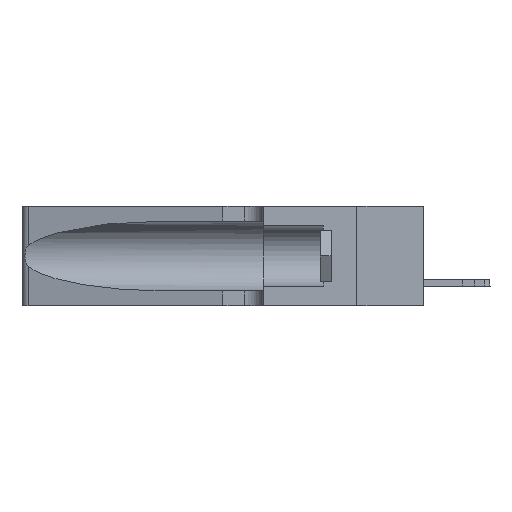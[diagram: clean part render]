
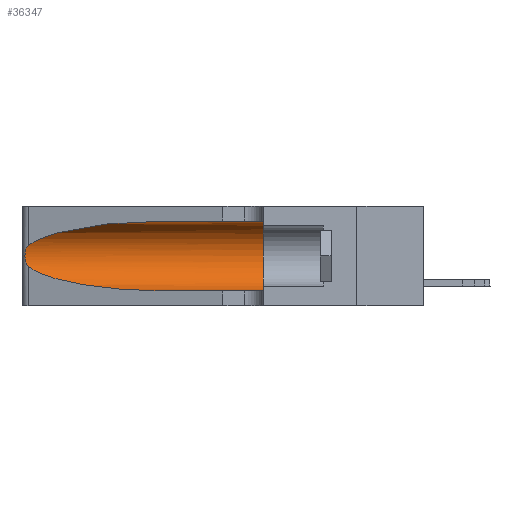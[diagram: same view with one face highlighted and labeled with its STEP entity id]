
A CAD part, left-side view. The second image highlights one B-rep face of the part: STEP entity #36347.
In plain terms, the highlighted cylindrical face has radius 3.308 mm (diameter 6.617 mm), a partial arc.
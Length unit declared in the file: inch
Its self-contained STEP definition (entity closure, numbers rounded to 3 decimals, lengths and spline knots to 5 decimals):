
#1433 = VECTOR ( 'NONE', #16997, 39.37008 ) ;
#1900 = ORIENTED_EDGE ( 'NONE', *, *, #30829, .F. ) ;
#3373 =( BOUNDED_CURVE ( )  B_SPLINE_CURVE ( 3, ( #14311, #23083, #34275, #22967 ),
 .UNSPECIFIED., .F., .F. ) 
 B_SPLINE_CURVE_WITH_KNOTS ( ( 4, 4 ),
 ( 1.5708, 2.84003 ),
 .UNSPECIFIED. ) 
 CURVE ( )  GEOMETRIC_REPRESENTATION_ITEM ( )  RATIONAL_B_SPLINE_CURVE ( ( 1., 0.87, 0.87, 1. ) ) 
 REPRESENTATION_ITEM ( '' )  );
#4114 = LINE ( 'NONE', #8895, #1433 ) ;
#4360 = CARTESIAN_POINT ( 'NONE',  ( 0.25639, 1.23184, 0.21858 ) ) ;
#4485 = CARTESIAN_POINT ( 'NONE',  ( 0.26075, 1.23896, 0.178 ) ) ;
#4694 = EDGE_CURVE ( 'NONE', #17199, #26774, #3373, .T. ) ;
#6088 = B_SPLINE_CURVE_WITH_KNOTS ( 'NONE', 3,
 ( #10452, #27189, #4360, #35996, #30304, #21318, #24179, #4485, #7190, #27065, #10196, #30049, #16656, #16875 ),
 .UNSPECIFIED., .F., .F.,
 ( 4, 2, 2, 2, 2, 2, 4 ),
 ( 0., 0.00027, 0.00053, 0.00107, 0.0016, 0.00187, 0.00214 ),
 .UNSPECIFIED. ) ;
#6370 = CARTESIAN_POINT ( 'NONE',  ( 0.1305, 0.72297, 0.05475 ) ) ;
#6477 = VECTOR ( 'NONE', #21810, 39.37008 ) ;
#7190 = CARTESIAN_POINT ( 'NONE',  ( 0.26017, 1.23833, 0.17102 ) ) ;
#7829 = CARTESIAN_POINT ( 'NONE',  ( 0.25487, 1.22718, 0.22369 ) ) ;
#8705 = CARTESIAN_POINT ( 'NONE',  ( 0.1305, 0.72297, 0.05475 ) ) ;
#8895 = CARTESIAN_POINT ( 'NONE',  ( 0.1305, 1.61858, 0.05475 ) ) ;
#9592 = FACE_OUTER_BOUND ( 'NONE', #34367, .T. ) ;
#10196 = CARTESIAN_POINT ( 'NONE',  ( 0.25789, 1.23486, 0.15765 ) ) ;
#10452 = CARTESIAN_POINT ( 'NONE',  ( 0.25487, 1.22718, 0.22369 ) ) ;
#11776 = LINE ( 'NONE', #21681, #6477 ) ;
#13000 = VERTEX_POINT ( 'NONE', #6370 ) ;
#13904 = VERTEX_POINT ( 'NONE', #18383 ) ;
#14230 = EDGE_CURVE ( 'NONE', #26774, #32012, #6088, .T. ) ;
#14311 = CARTESIAN_POINT ( 'NONE',  ( 0.1305, 0.72297, 0.31525 ) ) ;
#15037 = DIRECTION ( 'NONE',  ( 0., 1., 0. ) ) ;
#15459 = CARTESIAN_POINT ( 'NONE',  ( 0.1305, 0.72297, 0.31525 ) ) ;
#15637 = AXIS2_PLACEMENT_3D ( 'NONE', #34630, #15037, #34880 ) ;
#16471 = CARTESIAN_POINT ( 'NONE',  ( 0.1305, 0.35, 0.05475 ) ) ;
#16603 =( BOUNDED_CURVE ( )  B_SPLINE_CURVE ( 3, ( #20104, #31654, #28790, #8705 ),
 .UNSPECIFIED., .F., .T. ) 
 B_SPLINE_CURVE_WITH_KNOTS ( ( 4, 4 ),
 ( 3.44316, 4.71239 ),
 .UNSPECIFIED. ) 
 CURVE ( )  GEOMETRIC_REPRESENTATION_ITEM ( )  RATIONAL_B_SPLINE_CURVE ( ( 1., 0.87, 0.87, 1. ) ) 
 REPRESENTATION_ITEM ( '' )  );
#16656 = CARTESIAN_POINT ( 'NONE',  ( 0.25555, 1.22993, 0.14849 ) ) ;
#16875 = CARTESIAN_POINT ( 'NONE',  ( 0.25487, 1.22718, 0.14631 ) ) ;
#16913 = ORIENTED_EDGE ( 'NONE', *, *, #22742, .T. ) ;
#16997 = DIRECTION ( 'NONE',  ( 0., -1., 0. ) ) ;
#17199 = VERTEX_POINT ( 'NONE', #15459 ) ;
#17333 = DIRECTION ( 'NONE',  ( 0., -1., 0. ) ) ;
#18383 = CARTESIAN_POINT ( 'NONE',  ( 0.1305, 0.35, 0.31525 ) ) ;
#18998 = CIRCLE ( 'NONE', #15637, 0.13025 ) ;
#19406 = ORIENTED_EDGE ( 'NONE', *, *, #4694, .T. ) ;
#19585 = VERTEX_POINT ( 'NONE', #16471 ) ;
#20104 = CARTESIAN_POINT ( 'NONE',  ( 0.25487, 1.22718, 0.14631 ) ) ;
#20438 = AXIS2_PLACEMENT_3D ( 'NONE', #22058, #17333, #25766 ) ;
#21318 = CARTESIAN_POINT ( 'NONE',  ( 0.26018, 1.23835, 0.19895 ) ) ;
#21329 = ORIENTED_EDGE ( 'NONE', *, *, #31750, .T. ) ;
#21681 = CARTESIAN_POINT ( 'NONE',  ( 0.1305, 1.61858, 0.31525 ) ) ;
#21810 = DIRECTION ( 'NONE',  ( 0., -1., 0. ) ) ;
#22058 = CARTESIAN_POINT ( 'NONE',  ( 0.1305, 1.61858, 0.185 ) ) ;
#22742 = EDGE_CURVE ( 'NONE', #13000, #19585, #4114, .T. ) ;
#22967 = CARTESIAN_POINT ( 'NONE',  ( 0.25487, 1.22718, 0.22369 ) ) ;
#23083 = CARTESIAN_POINT ( 'NONE',  ( 0.18966, 0.96281, 0.31525 ) ) ;
#24179 = CARTESIAN_POINT ( 'NONE',  ( 0.26075, 1.23896, 0.19203 ) ) ;
#25766 = DIRECTION ( 'NONE',  ( 0., 0., -1. ) ) ;
#26155 = EDGE_CURVE ( 'NONE', #13904, #19585, #18998, .T. ) ;
#26774 = VERTEX_POINT ( 'NONE', #7829 ) ;
#27065 = CARTESIAN_POINT ( 'NONE',  ( 0.25856, 1.23593, 0.16098 ) ) ;
#27189 = CARTESIAN_POINT ( 'NONE',  ( 0.25555, 1.22994, 0.2215 ) ) ;
#27289 = ORIENTED_EDGE ( 'NONE', *, *, #14230, .T. ) ;
#28790 = CARTESIAN_POINT ( 'NONE',  ( 0.18966, 0.96281, 0.05475 ) ) ;
#29935 = ORIENTED_EDGE ( 'NONE', *, *, #26155, .F. ) ;
#30049 = CARTESIAN_POINT ( 'NONE',  ( 0.25639, 1.23186, 0.15144 ) ) ;
#30304 = CARTESIAN_POINT ( 'NONE',  ( 0.25854, 1.2359, 0.20912 ) ) ;
#30402 = CARTESIAN_POINT ( 'NONE',  ( 0.25487, 1.22718, 0.14631 ) ) ;
#30829 = EDGE_CURVE ( 'NONE', #17199, #13904, #11776, .T. ) ;
#31654 = CARTESIAN_POINT ( 'NONE',  ( 0.2373, 1.15595, 0.08982 ) ) ;
#31750 = EDGE_CURVE ( 'NONE', #32012, #13000, #16603, .T. ) ;
#32012 = VERTEX_POINT ( 'NONE', #30402 ) ;
#34275 = CARTESIAN_POINT ( 'NONE',  ( 0.2373, 1.15595, 0.28018 ) ) ;
#34367 = EDGE_LOOP ( 'NONE', ( #19406, #27289, #21329, #16913, #29935, #1900 ) ) ;
#34630 = CARTESIAN_POINT ( 'NONE',  ( 0.1305, 0.35, 0.185 ) ) ;
#34880 = DIRECTION ( 'NONE',  ( 0., 0., 1. ) ) ;
#35996 = CARTESIAN_POINT ( 'NONE',  ( 0.25787, 1.23484, 0.2124 ) ) ;
#36261 = CYLINDRICAL_SURFACE ( 'NONE', #20438, 0.13025 ) ;
#36347 = ADVANCED_FACE ( 'NONE', ( #9592 ), #36261, .F. ) ;
